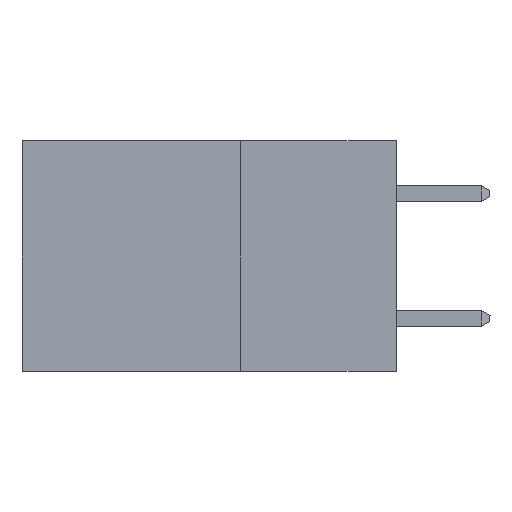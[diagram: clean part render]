
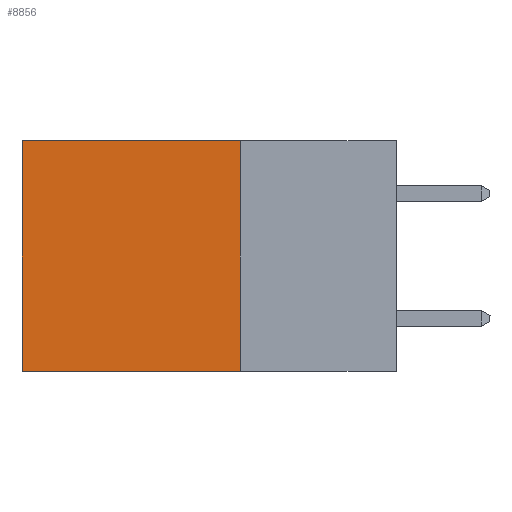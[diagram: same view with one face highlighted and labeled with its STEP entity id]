
A CAD part, left-side view. The second image highlights one B-rep face of the part: STEP entity #8856.
In plain terms, the highlighted planar face has unit normal (-1, 0, 0).
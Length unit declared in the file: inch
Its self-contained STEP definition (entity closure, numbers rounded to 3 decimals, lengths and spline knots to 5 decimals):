
#98 = VECTOR ( 'NONE', #9108, 39.37008 ) ;
#1136 = PLANE ( 'NONE',  #12403 ) ;
#1560 = LINE ( 'NONE', #5972, #6906 ) ;
#2970 = ORIENTED_EDGE ( 'NONE', *, *, #13153, .T. ) ;
#3323 = DIRECTION ( 'NONE',  ( 1., 0., 0. ) ) ;
#3482 = ORIENTED_EDGE ( 'NONE', *, *, #9590, .T. ) ;
#3529 = CARTESIAN_POINT ( 'NONE',  ( 0.2615, 0.25, 0. ) ) ;
#3636 = LINE ( 'NONE', #3916, #98 ) ;
#3916 = CARTESIAN_POINT ( 'NONE',  ( 0.2615, 0.25, -0.37 ) ) ;
#3951 = LINE ( 'NONE', #12584, #11195 ) ;
#5074 = VERTEX_POINT ( 'NONE', #9948 ) ;
#5368 = VERTEX_POINT ( 'NONE', #8391 ) ;
#5553 = DIRECTION ( 'NONE',  ( 0., 1., 0. ) ) ;
#5972 = CARTESIAN_POINT ( 'NONE',  ( 0.2615, 0.25, -0.37 ) ) ;
#6177 = VERTEX_POINT ( 'NONE', #3529 ) ;
#6184 = EDGE_LOOP ( 'NONE', ( #2970, #13241, #13006, #3482 ) ) ;
#6829 = FACE_OUTER_BOUND ( 'NONE', #6184, .T. ) ;
#6906 = VECTOR ( 'NONE', #11042, 39.37008 ) ;
#7339 = CARTESIAN_POINT ( 'NONE',  ( 0.2615, 0.6, 0. ) ) ;
#7504 = VERTEX_POINT ( 'NONE', #7339 ) ;
#8105 = VECTOR ( 'NONE', #5553, 39.37008 ) ;
#8391 = CARTESIAN_POINT ( 'NONE',  ( 0.2615, 0.6, -0.37 ) ) ;
#8571 = CARTESIAN_POINT ( 'NONE',  ( 0.2615, 0.25, -0.37 ) ) ;
#8856 = ADVANCED_FACE ( 'NONE', ( #6829 ), #1136, .F. ) ;
#9108 = DIRECTION ( 'NONE',  ( 0., 1., 0. ) ) ;
#9590 = EDGE_CURVE ( 'NONE', #6177, #7504, #11067, .T. ) ;
#9948 = CARTESIAN_POINT ( 'NONE',  ( 0.2615, 0.25, -0.37 ) ) ;
#10568 = DIRECTION ( 'NONE',  ( 0., 0., -1. ) ) ;
#10636 = CARTESIAN_POINT ( 'NONE',  ( 0.2615, 0.25, 0. ) ) ;
#10645 = DIRECTION ( 'NONE',  ( 0., 0., -1. ) ) ;
#11042 = DIRECTION ( 'NONE',  ( 0., 0., -1. ) ) ;
#11067 = LINE ( 'NONE', #10636, #8105 ) ;
#11195 = VECTOR ( 'NONE', #10645, 39.37008 ) ;
#11676 = EDGE_CURVE ( 'NONE', #6177, #5074, #1560, .T. ) ;
#12340 = EDGE_CURVE ( 'NONE', #5074, #5368, #3636, .T. ) ;
#12403 = AXIS2_PLACEMENT_3D ( 'NONE', #8571, #3323, #10568 ) ;
#12584 = CARTESIAN_POINT ( 'NONE',  ( 0.2615, 0.6, -0.37 ) ) ;
#13006 = ORIENTED_EDGE ( 'NONE', *, *, #11676, .F. ) ;
#13153 = EDGE_CURVE ( 'NONE', #7504, #5368, #3951, .T. ) ;
#13241 = ORIENTED_EDGE ( 'NONE', *, *, #12340, .F. ) ;
